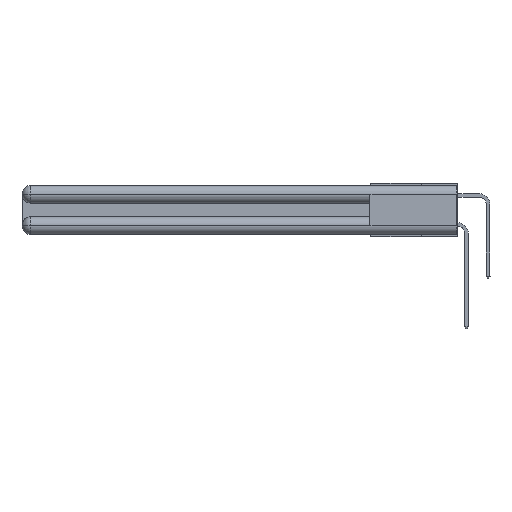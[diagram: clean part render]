
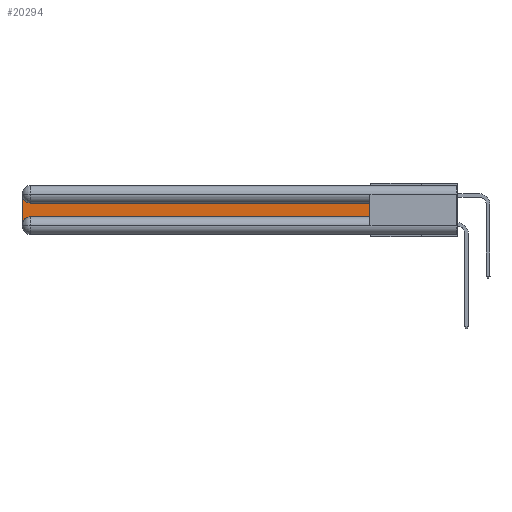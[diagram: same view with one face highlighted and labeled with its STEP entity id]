
A CAD part, left-side view. The second image highlights one B-rep face of the part: STEP entity #20294.
In plain terms, the highlighted planar face has unit normal (-1, 0, 0).
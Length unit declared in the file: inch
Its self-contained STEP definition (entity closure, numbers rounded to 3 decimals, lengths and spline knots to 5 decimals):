
#2231 = CARTESIAN_POINT ( 'NONE',  ( 0.075, 0.6, -0.2175 ) ) ;
#2564 = CIRCLE ( 'NONE', #10652, 0.06 ) ;
#2859 = EDGE_CURVE ( 'NONE', #31029, #30580, #10807, .T. ) ;
#3786 = CARTESIAN_POINT ( 'NONE',  ( 0.075, 2.94, -0.0625 ) ) ;
#5154 = ORIENTED_EDGE ( 'NONE', *, *, #26872, .T. ) ;
#6010 = EDGE_CURVE ( 'NONE', #21688, #31029, #16407, .T. ) ;
#6176 = DIRECTION ( 'NONE',  ( 1., 0., 0. ) ) ;
#7439 = DIRECTION ( 'NONE',  ( 0., 0., -1. ) ) ;
#8594 = ORIENTED_EDGE ( 'NONE', *, *, #20512, .T. ) ;
#9140 = EDGE_CURVE ( 'NONE', #22646, #31563, #10011, .T. ) ;
#9514 = DIRECTION ( 'NONE',  ( 0., 0., 1. ) ) ;
#9754 = VECTOR ( 'NONE', #9514, 39.37008 ) ;
#10011 = LINE ( 'NONE', #27015, #17027 ) ;
#10323 = EDGE_CURVE ( 'NONE', #30580, #22646, #2564, .T. ) ;
#10652 = AXIS2_PLACEMENT_3D ( 'NONE', #3786, #6176, #13609 ) ;
#10807 = LINE ( 'NONE', #16001, #15861 ) ;
#11745 = CARTESIAN_POINT ( 'NONE',  ( 0.075, 2.94, -0.2175 ) ) ;
#12144 = DIRECTION ( 'NONE',  ( 0., -1., 0. ) ) ;
#13609 = DIRECTION ( 'NONE',  ( 0., 0., -1. ) ) ;
#13617 = ORIENTED_EDGE ( 'NONE', *, *, #10323, .T. ) ;
#13623 = DIRECTION ( 'NONE',  ( 0., 1., 0. ) ) ;
#13751 = AXIS2_PLACEMENT_3D ( 'NONE', #25182, #27611, #7439 ) ;
#15861 = VECTOR ( 'NONE', #13623, 39.37008 ) ;
#16001 = CARTESIAN_POINT ( 'NONE',  ( 0.075, 0.6, -0.1225 ) ) ;
#16052 = CARTESIAN_POINT ( 'NONE',  ( 0.075, 2.94, -0.1225 ) ) ;
#16407 = LINE ( 'NONE', #24819, #9754 ) ;
#17027 = VECTOR ( 'NONE', #29445, 39.37008 ) ;
#17611 = PLANE ( 'NONE',  #28882 ) ;
#17889 = ORIENTED_EDGE ( 'NONE', *, *, #6010, .T. ) ;
#18509 = CARTESIAN_POINT ( 'NONE',  ( 0.075, 0.6, -0.1225 ) ) ;
#19830 = FACE_OUTER_BOUND ( 'NONE', #20028, .T. ) ;
#19944 = CARTESIAN_POINT ( 'NONE',  ( 0.075, 0.6, -0.2175 ) ) ;
#20028 = EDGE_LOOP ( 'NONE', ( #23263, #13617, #27343, #8594, #5154, #17889 ) ) ;
#20208 = DIRECTION ( 'NONE',  ( 0., 0., -1. ) ) ;
#20294 = ADVANCED_FACE ( 'NONE', ( #19830 ), #17611, .F. ) ;
#20321 = DIRECTION ( 'NONE',  ( 1., 0., 0. ) ) ;
#20512 = EDGE_CURVE ( 'NONE', #31563, #31124, #30884, .T. ) ;
#21492 = CARTESIAN_POINT ( 'NONE',  ( 0.075, 3., -0.0625 ) ) ;
#21688 = VERTEX_POINT ( 'NONE', #19944 ) ;
#22646 = VERTEX_POINT ( 'NONE', #21492 ) ;
#23090 = CARTESIAN_POINT ( 'NONE',  ( 0.075, 3., -0.1225 ) ) ;
#23263 = ORIENTED_EDGE ( 'NONE', *, *, #2859, .T. ) ;
#23599 = LINE ( 'NONE', #2231, #24735 ) ;
#24735 = VECTOR ( 'NONE', #12144, 39.37008 ) ;
#24819 = CARTESIAN_POINT ( 'NONE',  ( 0.075, 0.6, -0.2175 ) ) ;
#25182 = CARTESIAN_POINT ( 'NONE',  ( 0.075, 2.94, -0.2775 ) ) ;
#26872 = EDGE_CURVE ( 'NONE', #31124, #21688, #23599, .T. ) ;
#27015 = CARTESIAN_POINT ( 'NONE',  ( 0.075, 3., -0.2175 ) ) ;
#27343 = ORIENTED_EDGE ( 'NONE', *, *, #9140, .T. ) ;
#27611 = DIRECTION ( 'NONE',  ( 1., 0., 0. ) ) ;
#28882 = AXIS2_PLACEMENT_3D ( 'NONE', #23090, #20321, #20208 ) ;
#29067 = CARTESIAN_POINT ( 'NONE',  ( 0.075, 3., -0.2775 ) ) ;
#29445 = DIRECTION ( 'NONE',  ( 0., 0., -1. ) ) ;
#30580 = VERTEX_POINT ( 'NONE', #16052 ) ;
#30884 = CIRCLE ( 'NONE', #13751, 0.06 ) ;
#31029 = VERTEX_POINT ( 'NONE', #18509 ) ;
#31124 = VERTEX_POINT ( 'NONE', #11745 ) ;
#31563 = VERTEX_POINT ( 'NONE', #29067 ) ;
